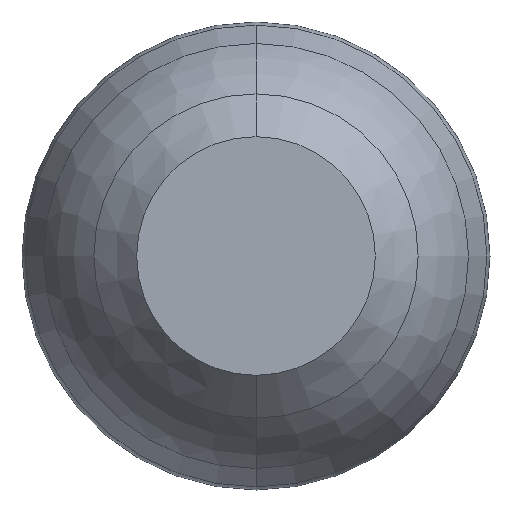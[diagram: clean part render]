
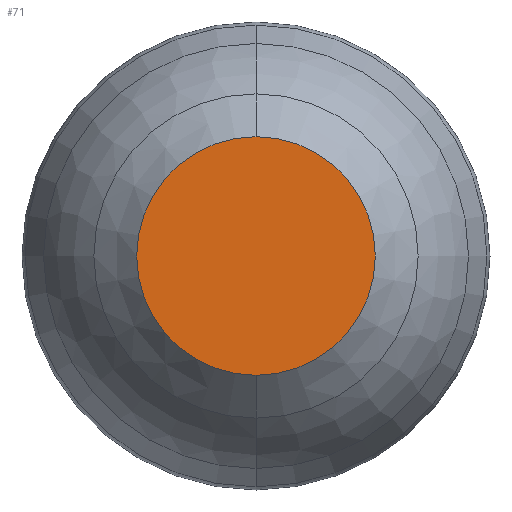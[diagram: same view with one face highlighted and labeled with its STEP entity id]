
A CAD part, front view. The second image highlights one B-rep face of the part: STEP entity #71.
In plain terms, the highlighted planar face has unit normal (0, -1, 0).
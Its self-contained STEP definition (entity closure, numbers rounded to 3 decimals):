
#10 = CARTESIAN_POINT ( 'NONE',  ( 0., -5., 0. ) ) ;
#11 = EDGE_CURVE ( 'NONE', #318, #350, #222, .T. ) ;
#12 = DIRECTION ( 'NONE',  ( 0., -1., 0. ) ) ;
#31 = CARTESIAN_POINT ( 'NONE',  ( 0., -5., -2.625 ) ) ;
#67 = CARTESIAN_POINT ( 'NONE',  ( 0., -5., 2.625 ) ) ;
#71 = ADVANCED_FACE ( 'NONE', ( #194 ), #366, .T. ) ;
#131 = CIRCLE ( 'NONE', #280, 2.625 ) ;
#192 = AXIS2_PLACEMENT_3D ( 'NONE', #365, #356, #328 ) ;
#194 = FACE_OUTER_BOUND ( 'NONE', #207, .T. ) ;
#207 = EDGE_LOOP ( 'NONE', ( #298, #299 ) ) ;
#222 = CIRCLE ( 'NONE', #370, 2.625 ) ;
#280 = AXIS2_PLACEMENT_3D ( 'NONE', #10, #12, #387 ) ;
#298 = ORIENTED_EDGE ( 'NONE', *, *, #11, .T. ) ;
#299 = ORIENTED_EDGE ( 'NONE', *, *, #345, .T. ) ;
#318 = VERTEX_POINT ( 'NONE', #67 ) ;
#328 = DIRECTION ( 'NONE',  ( 0., 0., -1. ) ) ;
#340 = CARTESIAN_POINT ( 'NONE',  ( 0., -5., 0. ) ) ;
#345 = EDGE_CURVE ( 'NONE', #350, #318, #131, .T. ) ;
#350 = VERTEX_POINT ( 'NONE', #31 ) ;
#356 = DIRECTION ( 'NONE',  ( 0., -1., 0. ) ) ;
#365 = CARTESIAN_POINT ( 'NONE',  ( 0., -5., 0. ) ) ;
#366 = PLANE ( 'NONE',  #192 ) ;
#370 = AXIS2_PLACEMENT_3D ( 'NONE', #340, #417, #411 ) ;
#387 = DIRECTION ( 'NONE',  ( 0., 0., -1. ) ) ;
#411 = DIRECTION ( 'NONE',  ( 0., 0., -1. ) ) ;
#417 = DIRECTION ( 'NONE',  ( 0., -1., 0. ) ) ;
